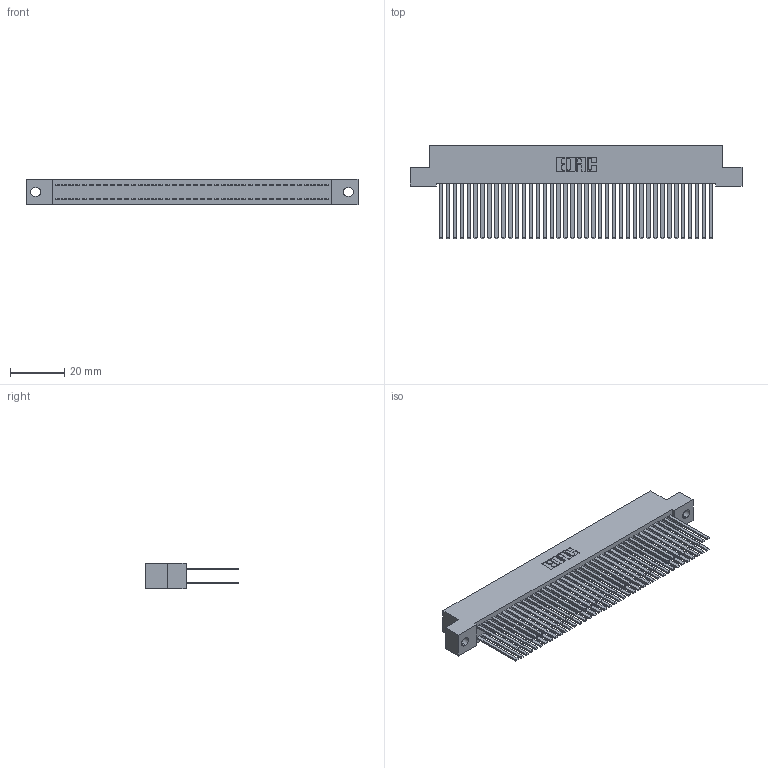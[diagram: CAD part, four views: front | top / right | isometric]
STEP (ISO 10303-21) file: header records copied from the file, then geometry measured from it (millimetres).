
FILE_DESCRIPTION (( 'STEP AP203' ), '1' );
FILE_NAME ('342-080-544-202.STEP', '2018-08-13T15:10:35', ( '' ), ( '' ), 'SwSTEP 2.0', 'SolidWorks 2016', '' );
FILE_SCHEMA (( 'CONFIG_CONTROL_DESIGN' ));
Length unit declared in the file: inch
Products named in the file (3): 342 Part_.128 Slot; 345-292-001_345-293-144; 342-080-544-202
Assembly tree (81 placements, depth 2):
  342-080-544-202
    342 Part_.128 Slot
    345-292-001_345-293-144  x80
Bounding box: 121.92 x 34.3 x 9.4 mm (x, y, z)
Volume: 12014.3 mm3; surface area: 22372.2 mm2
Topology: 81 solids, 81 shells, 3794 faces, 11271 edges, 7406 vertices
Faces by surface type: plane 2630, cylinder 1164
Entity records: 25811 total; most frequent: CARTESIAN_POINT 4278, ORIENTED_EDGE 4214, DIRECTION 3655, EDGE_CURVE 2107, LINE 1983, VECTOR 1983, VERTEX_POINT 1402, AXIS2_PLACEMENT_3D 836
